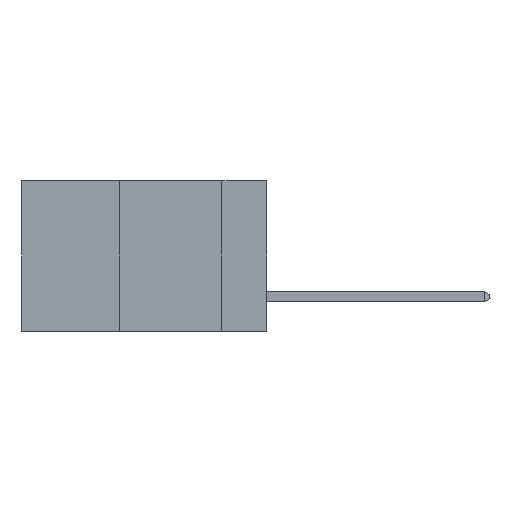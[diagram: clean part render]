
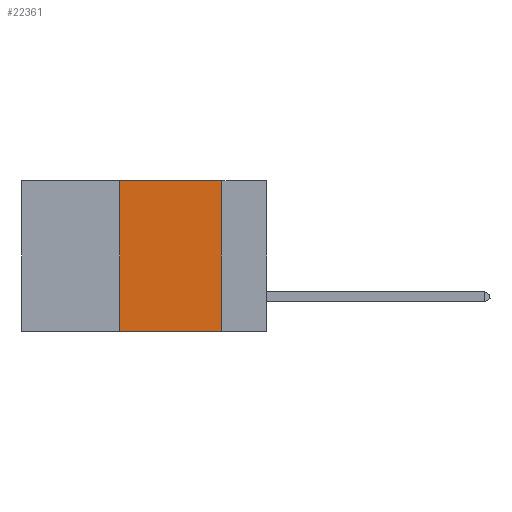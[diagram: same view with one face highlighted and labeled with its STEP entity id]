
A CAD part, left-side view. The second image highlights one B-rep face of the part: STEP entity #22361.
In plain terms, the highlighted planar face has unit normal (-1, 0, 0).
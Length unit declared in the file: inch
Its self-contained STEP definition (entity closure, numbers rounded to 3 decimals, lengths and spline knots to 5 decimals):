
#709 = CARTESIAN_POINT ( 'NONE',  ( 0., 0.36, -0.37 ) ) ;
#875 = DIRECTION ( 'NONE',  ( 0., -1., 0. ) ) ;
#1140 = EDGE_CURVE ( 'NONE', #4870, #15157, #21247, .T. ) ;
#1899 = VECTOR ( 'NONE', #18247, 39.37008 ) ;
#2077 = CARTESIAN_POINT ( 'NONE',  ( 0., 0.6, 0. ) ) ;
#2670 = PLANE ( 'NONE',  #22737 ) ;
#2862 = ORIENTED_EDGE ( 'NONE', *, *, #1140, .F. ) ;
#4870 = VERTEX_POINT ( 'NONE', #15464 ) ;
#5312 = DIRECTION ( 'NONE',  ( 0., 0., -1. ) ) ;
#5680 = VECTOR ( 'NONE', #20346, 39.37008 ) ;
#6556 = CARTESIAN_POINT ( 'NONE',  ( 0., 0.11, -0.37 ) ) ;
#6757 = DIRECTION ( 'NONE',  ( 1., 0., 0. ) ) ;
#9036 = EDGE_CURVE ( 'NONE', #19440, #4870, #22135, .T. ) ;
#10068 = ORIENTED_EDGE ( 'NONE', *, *, #9036, .F. ) ;
#11358 = CARTESIAN_POINT ( 'NONE',  ( 0., 0.11, 0. ) ) ;
#12011 = LINE ( 'NONE', #12601, #5680 ) ;
#12601 = CARTESIAN_POINT ( 'NONE',  ( 0., 0.36, 0. ) ) ;
#15157 = VERTEX_POINT ( 'NONE', #6556 ) ;
#15198 = VERTEX_POINT ( 'NONE', #709 ) ;
#15464 = CARTESIAN_POINT ( 'NONE',  ( 0., 0.11, 0. ) ) ;
#15627 = VECTOR ( 'NONE', #875, 39.37008 ) ;
#16193 = VECTOR ( 'NONE', #5312, 39.37008 ) ;
#16989 = EDGE_CURVE ( 'NONE', #15198, #19440, #12011, .T. ) ;
#17884 = CARTESIAN_POINT ( 'NONE',  ( 0., 0.36, 0. ) ) ;
#18247 = DIRECTION ( 'NONE',  ( 0., -1., 0. ) ) ;
#18831 = CARTESIAN_POINT ( 'NONE',  ( 0., 0.6, 0. ) ) ;
#19440 = VERTEX_POINT ( 'NONE', #17884 ) ;
#20346 = DIRECTION ( 'NONE',  ( 0., 0., 1. ) ) ;
#21247 = LINE ( 'NONE', #11358, #16193 ) ;
#21497 = ORIENTED_EDGE ( 'NONE', *, *, #16989, .F. ) ;
#21943 = EDGE_LOOP ( 'NONE', ( #2862, #10068, #21497, #25060 ) ) ;
#22135 = LINE ( 'NONE', #2077, #1899 ) ;
#22361 = ADVANCED_FACE ( 'NONE', ( #23870 ), #2670, .F. ) ;
#22737 = AXIS2_PLACEMENT_3D ( 'NONE', #18831, #6757, #22901 ) ;
#22901 = DIRECTION ( 'NONE',  ( 0., 0., -1. ) ) ;
#23870 = FACE_OUTER_BOUND ( 'NONE', #21943, .T. ) ;
#24696 = CARTESIAN_POINT ( 'NONE',  ( 0., 0.6, -0.37 ) ) ;
#25060 = ORIENTED_EDGE ( 'NONE', *, *, #25456, .T. ) ;
#25456 = EDGE_CURVE ( 'NONE', #15198, #15157, #26078, .T. ) ;
#26078 = LINE ( 'NONE', #24696, #15627 ) ;
